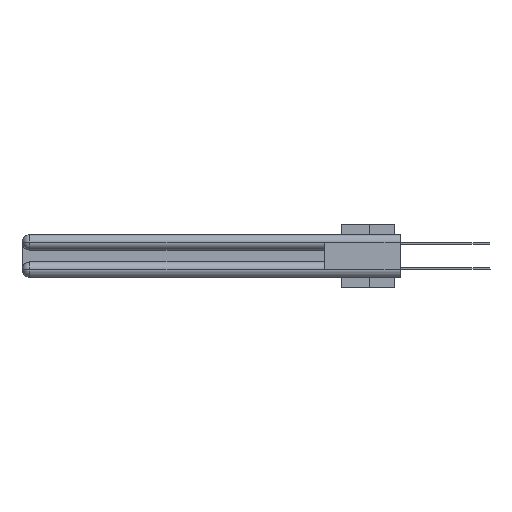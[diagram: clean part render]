
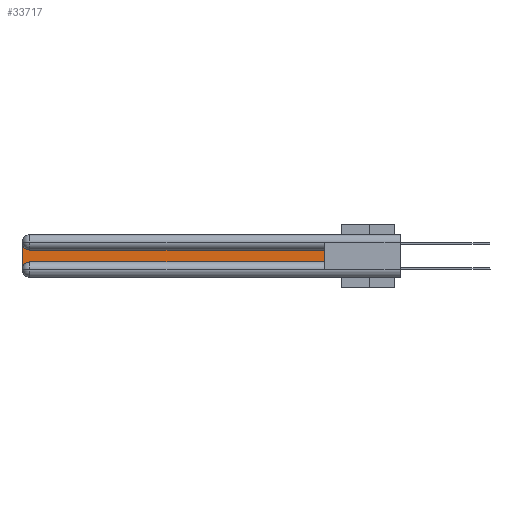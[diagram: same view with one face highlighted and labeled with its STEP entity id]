
A CAD part, left-side view. The second image highlights one B-rep face of the part: STEP entity #33717.
In plain terms, the highlighted planar face has unit normal (-1, 0, 0).
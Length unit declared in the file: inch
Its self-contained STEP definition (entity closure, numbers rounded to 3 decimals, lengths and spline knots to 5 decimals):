
#145 = AXIS2_PLACEMENT_3D ( 'NONE', #4130, #36827, #15644 ) ;
#2247 = VERTEX_POINT ( 'NONE', #28236 ) ;
#3639 = CARTESIAN_POINT ( 'NONE',  ( 0.075, 2.94, -0.0625 ) ) ;
#4130 = CARTESIAN_POINT ( 'NONE',  ( 0.075, 2.94, -0.2775 ) ) ;
#5533 = VERTEX_POINT ( 'NONE', #19682 ) ;
#6194 = ORIENTED_EDGE ( 'NONE', *, *, #9236, .T. ) ;
#6885 = EDGE_CURVE ( 'NONE', #5533, #9190, #20798, .T. ) ;
#7768 = CARTESIAN_POINT ( 'NONE',  ( 0.075, 3., -0.0625 ) ) ;
#9190 = VERTEX_POINT ( 'NONE', #16214 ) ;
#9236 = EDGE_CURVE ( 'NONE', #17364, #33898, #21945, .T. ) ;
#9724 = VECTOR ( 'NONE', #34499, 39.37008 ) ;
#9972 = FACE_OUTER_BOUND ( 'NONE', #18846, .T. ) ;
#10140 = CIRCLE ( 'NONE', #11390, 0.06 ) ;
#10419 = CARTESIAN_POINT ( 'NONE',  ( 0.075, 0.6, -0.2175 ) ) ;
#11390 = AXIS2_PLACEMENT_3D ( 'NONE', #3639, #15525, #19009 ) ;
#12904 = DIRECTION ( 'NONE',  ( 0., 0., -1. ) ) ;
#13505 = LINE ( 'NONE', #10419, #9724 ) ;
#14438 = ORIENTED_EDGE ( 'NONE', *, *, #15796, .T. ) ;
#14602 = DIRECTION ( 'NONE',  ( 0., 0., 1. ) ) ;
#14926 = ORIENTED_EDGE ( 'NONE', *, *, #29846, .T. ) ;
#15525 = DIRECTION ( 'NONE',  ( 1., 0., 0. ) ) ;
#15644 = DIRECTION ( 'NONE',  ( 0., 0., -1. ) ) ;
#15796 = EDGE_CURVE ( 'NONE', #2247, #5533, #38326, .T. ) ;
#16187 = VERTEX_POINT ( 'NONE', #7768 ) ;
#16214 = CARTESIAN_POINT ( 'NONE',  ( 0.075, 2.94, -0.1225 ) ) ;
#17364 = VERTEX_POINT ( 'NONE', #20509 ) ;
#17428 = AXIS2_PLACEMENT_3D ( 'NONE', #30944, #24547, #36219 ) ;
#18846 = EDGE_LOOP ( 'NONE', ( #27790, #23663, #14926, #6194, #38033, #14438 ) ) ;
#19009 = DIRECTION ( 'NONE',  ( 0., 0., -1. ) ) ;
#19682 = CARTESIAN_POINT ( 'NONE',  ( 0.075, 0.6, -0.1225 ) ) ;
#20509 = CARTESIAN_POINT ( 'NONE',  ( 0.075, 3., -0.2775 ) ) ;
#20798 = LINE ( 'NONE', #35951, #22501 ) ;
#21097 = CARTESIAN_POINT ( 'NONE',  ( 0.075, 3., -0.2175 ) ) ;
#21378 = DIRECTION ( 'NONE',  ( 0., 1., 0. ) ) ;
#21945 = CIRCLE ( 'NONE', #145, 0.06 ) ;
#22501 = VECTOR ( 'NONE', #21378, 39.37008 ) ;
#23663 = ORIENTED_EDGE ( 'NONE', *, *, #38152, .T. ) ;
#24354 = PLANE ( 'NONE',  #17428 ) ;
#24547 = DIRECTION ( 'NONE',  ( 1., 0., 0. ) ) ;
#27790 = ORIENTED_EDGE ( 'NONE', *, *, #6885, .T. ) ;
#28205 = EDGE_CURVE ( 'NONE', #33898, #2247, #13505, .T. ) ;
#28236 = CARTESIAN_POINT ( 'NONE',  ( 0.075, 0.6, -0.2175 ) ) ;
#29846 = EDGE_CURVE ( 'NONE', #16187, #17364, #33330, .T. ) ;
#30944 = CARTESIAN_POINT ( 'NONE',  ( 0.075, 3., -0.1225 ) ) ;
#32112 = CARTESIAN_POINT ( 'NONE',  ( 0.075, 0.6, -0.2175 ) ) ;
#32168 = VECTOR ( 'NONE', #14602, 39.37008 ) ;
#33330 = LINE ( 'NONE', #21097, #34054 ) ;
#33717 = ADVANCED_FACE ( 'NONE', ( #9972 ), #24354, .F. ) ;
#33898 = VERTEX_POINT ( 'NONE', #34822 ) ;
#34054 = VECTOR ( 'NONE', #12904, 39.37008 ) ;
#34499 = DIRECTION ( 'NONE',  ( 0., -1., 0. ) ) ;
#34822 = CARTESIAN_POINT ( 'NONE',  ( 0.075, 2.94, -0.2175 ) ) ;
#35951 = CARTESIAN_POINT ( 'NONE',  ( 0.075, 0.6, -0.1225 ) ) ;
#36219 = DIRECTION ( 'NONE',  ( 0., 0., -1. ) ) ;
#36827 = DIRECTION ( 'NONE',  ( 1., 0., 0. ) ) ;
#38033 = ORIENTED_EDGE ( 'NONE', *, *, #28205, .T. ) ;
#38152 = EDGE_CURVE ( 'NONE', #9190, #16187, #10140, .T. ) ;
#38326 = LINE ( 'NONE', #32112, #32168 ) ;
